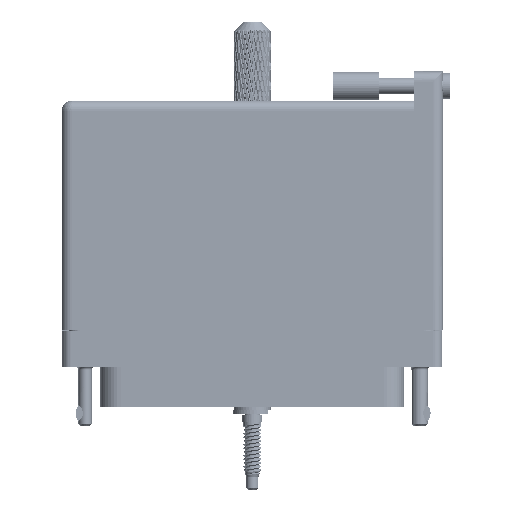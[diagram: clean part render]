
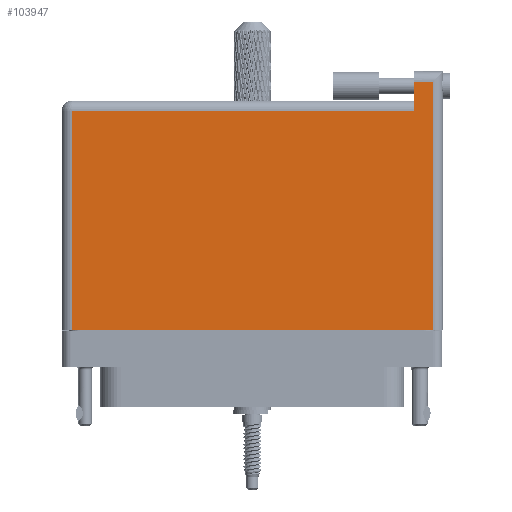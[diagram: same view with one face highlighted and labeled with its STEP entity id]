
A CAD part, front view. The second image highlights one B-rep face of the part: STEP entity #103947.
In plain terms, the highlighted face is planar.
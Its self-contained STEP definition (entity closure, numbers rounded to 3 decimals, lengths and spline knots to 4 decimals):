
#2207 = ORIENTED_EDGE ( 'NONE', *, *, #80627, .T. ) ;
#3132 = ORIENTED_EDGE ( 'NONE', *, *, #100639, .T. ) ;
#6168 = VECTOR ( 'NONE', #117912, 39.3701 ) ;
#8033 = CARTESIAN_POINT ( 'NONE',  ( -1.23, -0.1, 0.4495 ) ) ;
#9273 = DIRECTION ( 'NONE',  ( 1., 0., 0. ) ) ;
#12316 = DIRECTION ( 'NONE',  ( -1., 0., 0. ) ) ;
#18261 = LINE ( 'NONE', #77717, #65616 ) ;
#18380 = VECTOR ( 'NONE', #102151, 39.3701 ) ;
#20121 = AXIS2_PLACEMENT_3D ( 'NONE', #37562, #57226, #125643 ) ;
#20192 = VECTOR ( 'NONE', #67790, 39.3701 ) ;
#28096 = VERTEX_POINT ( 'NONE', #62747 ) ;
#28651 = EDGE_CURVE ( 'NONE', #79426, #122720, #122574, .T. ) ;
#34615 = CARTESIAN_POINT ( 'NONE',  ( 1.23, 1.596, 0.4495 ) ) ;
#37562 = CARTESIAN_POINT ( 'NONE',  ( -1.3, 1.466, 0.4495 ) ) ;
#38349 = EDGE_CURVE ( 'NONE', #122720, #74887, #106052, .T. ) ;
#38522 = CARTESIAN_POINT ( 'NONE',  ( 1.103, 1.596, 0.4495 ) ) ;
#41766 = VECTOR ( 'NONE', #9273, 39.3701 ) ;
#57060 = CARTESIAN_POINT ( 'NONE',  ( -1.3, -0.1, 0.4495 ) ) ;
#57226 = DIRECTION ( 'NONE',  ( 0., 0., -1. ) ) ;
#57411 = ORIENTED_EDGE ( 'NONE', *, *, #114553, .T. ) ;
#62747 = CARTESIAN_POINT ( 'NONE',  ( 1.103, 1.396, 0.4495 ) ) ;
#64089 = CARTESIAN_POINT ( 'NONE',  ( -1.23, 1.396, 0.4495 ) ) ;
#64157 = ORIENTED_EDGE ( 'NONE', *, *, #28651, .T. ) ;
#65616 = VECTOR ( 'NONE', #114360, 39.3701 ) ;
#67790 = DIRECTION ( 'NONE',  ( 0., -1., 0. ) ) ;
#68380 = EDGE_CURVE ( 'NONE', #79159, #28096, #18261, .T. ) ;
#73116 = ORIENTED_EDGE ( 'NONE', *, *, #38349, .T. ) ;
#74887 = VERTEX_POINT ( 'NONE', #91706 ) ;
#77717 = CARTESIAN_POINT ( 'NONE',  ( 1.103, 1.666, 0.4495 ) ) ;
#78347 = EDGE_LOOP ( 'NONE', ( #73116, #2207, #57411, #94371, #3132, #64157 ) ) ;
#79159 = VERTEX_POINT ( 'NONE', #38522 ) ;
#79426 = VERTEX_POINT ( 'NONE', #64089 ) ;
#80627 = EDGE_CURVE ( 'NONE', #74887, #92398, #113074, .T. ) ;
#81162 = LINE ( 'NONE', #91718, #110099 ) ;
#84174 = LINE ( 'NONE', #89284, #6168 ) ;
#86782 = PLANE ( 'NONE',  #20121 ) ;
#89284 = CARTESIAN_POINT ( 'NONE',  ( -1.3, 1.396, 0.4495 ) ) ;
#91706 = CARTESIAN_POINT ( 'NONE',  ( 1.23, -0.1, 0.4495 ) ) ;
#91718 = CARTESIAN_POINT ( 'NONE',  ( -1.3, 1.596, 0.4495 ) ) ;
#92398 = VERTEX_POINT ( 'NONE', #34615 ) ;
#94371 = ORIENTED_EDGE ( 'NONE', *, *, #68380, .T. ) ;
#95211 = CARTESIAN_POINT ( 'NONE',  ( -1.23, -0.1, 0.4495 ) ) ;
#100639 = EDGE_CURVE ( 'NONE', #28096, #79426, #84174, .T. ) ;
#102151 = DIRECTION ( 'NONE',  ( 0., 1., 0. ) ) ;
#103421 = CARTESIAN_POINT ( 'NONE',  ( 1.23, 1.666, 0.4495 ) ) ;
#103947 = ADVANCED_FACE ( 'NONE', ( #119981 ), #86782, .F. ) ;
#106052 = LINE ( 'NONE', #57060, #41766 ) ;
#110099 = VECTOR ( 'NONE', #12316, 39.3701 ) ;
#113074 = LINE ( 'NONE', #103421, #18380 ) ;
#114360 = DIRECTION ( 'NONE',  ( 0., -1., 0. ) ) ;
#114553 = EDGE_CURVE ( 'NONE', #92398, #79159, #81162, .T. ) ;
#117912 = DIRECTION ( 'NONE',  ( -1., 0., 0. ) ) ;
#119981 = FACE_OUTER_BOUND ( 'NONE', #78347, .T. ) ;
#122574 = LINE ( 'NONE', #8033, #20192 ) ;
#122720 = VERTEX_POINT ( 'NONE', #95211 ) ;
#125643 = DIRECTION ( 'NONE',  ( -1., 0., 0. ) ) ;
